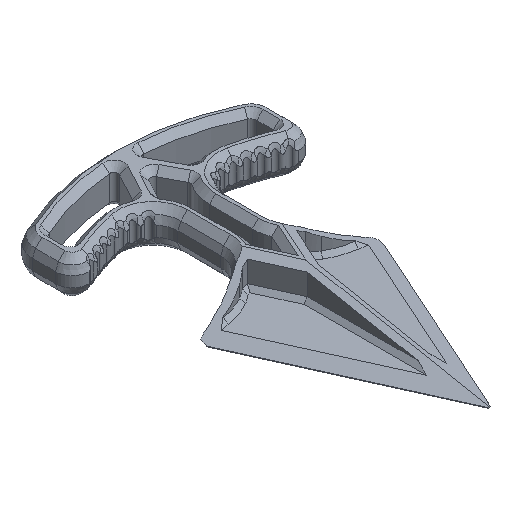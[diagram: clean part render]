
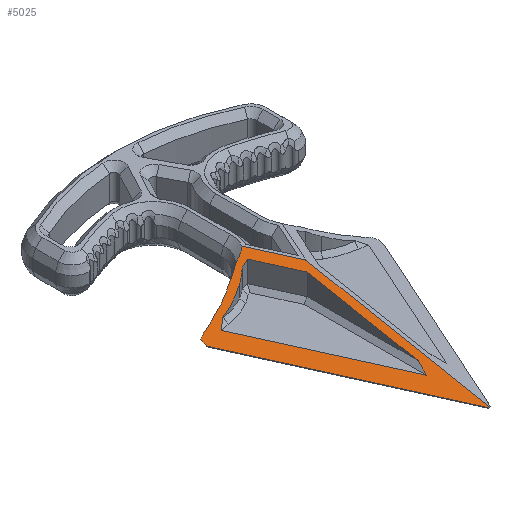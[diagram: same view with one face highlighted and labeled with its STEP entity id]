
A CAD part, isometric view. The second image highlights one B-rep face of the part: STEP entity #5025.
In plain terms, the highlighted planar face has unit normal (-0.385, -0.174, 0.906).
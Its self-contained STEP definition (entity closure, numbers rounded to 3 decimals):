
#60=ELLIPSE('',#5451,39.242,31.462);
#61=ELLIPSE('',#5458,33.593,30.446);
#62=ELLIPSE('',#5460,17.386,15.757);
#63=ELLIPSE('',#5462,13.645,12.367);
#64=ELLIPSE('',#5472,16.739,13.421);
#65=ELLIPSE('',#5475,8.311,6.663);
#66=ELLIPSE('',#5476,16.33,14.522);
#67=ELLIPSE('',#5477,16.084,14.577);
#68=ELLIPSE('',#5478,15.898,14.137);
#94=B_SPLINE_CURVE_WITH_KNOTS('',3,(#7758,#7759,#7760,#7761,#7762,#7763,
#7764,#7765,#7766,#7767,#7768,#7769,#7770),.UNSPECIFIED.,.F.,.F.,(4,3,3,
3,4),(0.053,0.072,0.09,0.104,
0.162),.UNSPECIFIED.);
#96=B_SPLINE_CURVE_WITH_KNOTS('',3,(#7791,#7792,#7793,#7794,#7795,#7796,
#7797),.UNSPECIFIED.,.F.,.F.,(4,3,4),(0.,0.045,0.053),
 .UNSPECIFIED.);
#335=FACE_BOUND('',#926,.T.);
#463=PLANE('',#5474);
#611=FACE_OUTER_BOUND('',#925,.T.);
#925=EDGE_LOOP('',(#3813,#3814,#3815,#3816,#3817,#3818,#3819,#3820,#3821,
#3822,#3823));
#926=EDGE_LOOP('',(#3824,#3825,#3826,#3827,#3828,#3829,#3830,#3831,#3832));
#1325=LINE('',#7068,#1644);
#1443=LINE('',#7509,#1762);
#1469=LINE('',#7636,#1788);
#1475=LINE('',#7653,#1794);
#1477=LINE('',#7657,#1796);
#1478=LINE('',#7659,#1797);
#1482=LINE('',#7669,#1801);
#1489=LINE('',#7700,#1808);
#1491=LINE('',#7809,#1810);
#1644=VECTOR('',#5796,10.);
#1762=VECTOR('',#6242,10.);
#1788=VECTOR('',#6338,10.);
#1794=VECTOR('',#6358,10.);
#1796=VECTOR('',#6362,10.);
#1797=VECTOR('',#6365,10.);
#1801=VECTOR('',#6371,10.);
#1808=VECTOR('',#6386,10.);
#1810=VECTOR('',#6396,10.);
#1970=VERTEX_POINT('',#7065);
#1971=VERTEX_POINT('',#7067);
#2104=VERTEX_POINT('',#7505);
#2106=VERTEX_POINT('',#7508);
#2133=VERTEX_POINT('',#7617);
#2136=VERTEX_POINT('',#7635);
#2137=VERTEX_POINT('',#7639);
#2138=VERTEX_POINT('',#7643);
#2139=VERTEX_POINT('',#7647);
#2140=VERTEX_POINT('',#7651);
#2141=VERTEX_POINT('',#7655);
#2145=VERTEX_POINT('',#7666);
#2146=VERTEX_POINT('',#7668);
#2151=VERTEX_POINT('',#7699);
#2154=VERTEX_POINT('',#7751);
#2156=VERTEX_POINT('',#7757);
#2157=VERTEX_POINT('',#7803);
#2159=VERTEX_POINT('',#7810);
#2160=VERTEX_POINT('',#7812);
#2161=VERTEX_POINT('',#7814);
#2466=EDGE_CURVE('',#1971,#1970,#1325,.T.);
#2678=EDGE_CURVE('',#2106,#2104,#1443,.T.);
#2719=EDGE_CURVE('',#2133,#2104,#60,.T.);
#2726=EDGE_CURVE('',#2106,#2136,#1469,.T.);
#2729=EDGE_CURVE('',#2133,#2137,#61,.T.);
#2731=EDGE_CURVE('',#2137,#2138,#62,.T.);
#2733=EDGE_CURVE('',#2138,#2139,#63,.T.);
#2735=EDGE_CURVE('',#2139,#2140,#1475,.T.);
#2737=EDGE_CURVE('',#2140,#2141,#1477,.T.);
#2738=EDGE_CURVE('',#2141,#2136,#1478,.T.);
#2742=EDGE_CURVE('',#2145,#2146,#1482,.T.);
#2752=EDGE_CURVE('',#2151,#2146,#1489,.T.);
#2758=EDGE_CURVE('',#2154,#2156,#94,.T.);
#2760=EDGE_CURVE('',#2151,#2154,#96,.T.);
#2762=EDGE_CURVE('',#2157,#2156,#64,.T.);
#2765=EDGE_CURVE('',#2145,#1971,#1491,.T.);
#2766=EDGE_CURVE('',#1970,#2159,#65,.T.);
#2767=EDGE_CURVE('',#2159,#2160,#66,.T.);
#2768=EDGE_CURVE('',#2160,#2161,#67,.T.);
#2769=EDGE_CURVE('',#2161,#2157,#68,.T.);
#3813=ORIENTED_EDGE('',*,*,#2742,.F.);
#3814=ORIENTED_EDGE('',*,*,#2765,.T.);
#3815=ORIENTED_EDGE('',*,*,#2466,.T.);
#3816=ORIENTED_EDGE('',*,*,#2766,.T.);
#3817=ORIENTED_EDGE('',*,*,#2767,.T.);
#3818=ORIENTED_EDGE('',*,*,#2768,.T.);
#3819=ORIENTED_EDGE('',*,*,#2769,.T.);
#3820=ORIENTED_EDGE('',*,*,#2762,.T.);
#3821=ORIENTED_EDGE('',*,*,#2758,.F.);
#3822=ORIENTED_EDGE('',*,*,#2760,.F.);
#3823=ORIENTED_EDGE('',*,*,#2752,.T.);
#3824=ORIENTED_EDGE('',*,*,#2738,.T.);
#3825=ORIENTED_EDGE('',*,*,#2726,.F.);
#3826=ORIENTED_EDGE('',*,*,#2678,.T.);
#3827=ORIENTED_EDGE('',*,*,#2719,.F.);
#3828=ORIENTED_EDGE('',*,*,#2729,.T.);
#3829=ORIENTED_EDGE('',*,*,#2731,.T.);
#3830=ORIENTED_EDGE('',*,*,#2733,.T.);
#3831=ORIENTED_EDGE('',*,*,#2735,.T.);
#3832=ORIENTED_EDGE('',*,*,#2737,.T.);
#5025=ADVANCED_FACE('',(#611,#335),#463,.T.);
#5451=AXIS2_PLACEMENT_3D('',#7619,#6322,#6323);
#5458=AXIS2_PLACEMENT_3D('',#7641,#6343,#6344);
#5460=AXIS2_PLACEMENT_3D('',#7645,#6348,#6349);
#5462=AXIS2_PLACEMENT_3D('',#7649,#6353,#6354);
#5472=AXIS2_PLACEMENT_3D('',#7804,#6389,#6390);
#5474=AXIS2_PLACEMENT_3D('',#7808,#6394,#6395);
#5475=AXIS2_PLACEMENT_3D('',#7811,#6397,#6398);
#5476=AXIS2_PLACEMENT_3D('',#7813,#6399,#6400);
#5477=AXIS2_PLACEMENT_3D('',#7815,#6401,#6402);
#5478=AXIS2_PLACEMENT_3D('',#7816,#6403,#6404);
#5796=DIRECTION('',(-0.411,0.911,0.));
#6242=DIRECTION('',(-0.411,0.911,0.));
#6322=DIRECTION('center_axis',(0.385,0.174,-0.906));
#6323=DIRECTION('ref_axis',(0.826,0.373,0.423));
#6338=DIRECTION('',(0.302,0.904,0.302));
#6343=DIRECTION('center_axis',(-0.385,-0.174,0.906));
#6344=DIRECTION('ref_axis',(-0.826,-0.373,-0.423));
#6348=DIRECTION('center_axis',(-0.385,-0.174,0.906));
#6349=DIRECTION('ref_axis',(-0.826,-0.373,-0.423));
#6353=DIRECTION('center_axis',(-0.385,-0.174,0.906));
#6354=DIRECTION('ref_axis',(0.826,0.373,0.423));
#6358=DIRECTION('',(0.879,0.23,0.418));
#6362=DIRECTION('',(0.411,-0.911,0.));
#6365=DIRECTION('',(0.,-0.982,-0.188));
#6371=DIRECTION('',(-0.92,0.,-0.391));
#6386=DIRECTION('',(0.411,-0.911,0.));
#6389=DIRECTION('center_axis',(0.385,0.174,-0.906));
#6390=DIRECTION('ref_axis',(0.826,0.373,0.423));
#6394=DIRECTION('center_axis',(-0.385,-0.174,0.906));
#6395=DIRECTION('ref_axis',(0.92,0.,0.391));
#6396=DIRECTION('',(0.,0.982,0.188));
#6397=DIRECTION('center_axis',(0.385,0.174,-0.906));
#6398=DIRECTION('ref_axis',(0.826,0.373,0.423));
#6399=DIRECTION('center_axis',(0.385,0.174,-0.906));
#6400=DIRECTION('ref_axis',(0.826,0.373,0.423));
#6401=DIRECTION('center_axis',(0.385,0.174,-0.906));
#6402=DIRECTION('ref_axis',(-0.826,-0.373,-0.423));
#6403=DIRECTION('center_axis',(0.385,0.174,-0.906));
#6404=DIRECTION('ref_axis',(0.826,0.373,0.423));
#7065=CARTESIAN_POINT('',(-4.712,-31.269,9.));
#7067=CARTESIAN_POINT('',(0.,-41.71,9.));
#7068=CARTESIAN_POINT('',(1.895,-45.908,9.));
#7505=CARTESIAN_POINT('',(-17.632,-39.134,2.));
#7508=CARTESIAN_POINT('',(-2.4,-72.884,2.));
#7509=CARTESIAN_POINT('',(-10.949,-53.941,2.));
#7617=CARTESIAN_POINT('',(-15.904,-37.75,3.));
#7619=CARTESIAN_POINT('Origin',(-38.221,-14.991,-2.119));
#7635=CARTESIAN_POINT('',(-1.4,-69.886,3.));
#7636=CARTESIAN_POINT('',(3.643,-54.771,8.043));
#7639=CARTESIAN_POINT('',(-15.7,-37.7,3.096));
#7641=CARTESIAN_POINT('Origin',(-23.105,-8.168,5.614));
#7643=CARTESIAN_POINT('',(-9.695,-35.648,6.042));
#7645=CARTESIAN_POINT('Origin',(-17.688,-22.069,5.25));
#7647=CARTESIAN_POINT('',(-7.517,-34.042,7.276));
#7649=CARTESIAN_POINT('Origin',(-15.901,-24.951,5.457));
#7651=CARTESIAN_POINT('',(-5.852,-33.606,8.067));
#7653=CARTESIAN_POINT('',(-9.498,-34.562,6.334));
#7655=CARTESIAN_POINT('',(-1.4,-43.47,8.067));
#7657=CARTESIAN_POINT('',(-1.023,-44.304,8.067));
#7659=CARTESIAN_POINT('',(-1.4,-51.311,6.563));
#7666=CARTESIAN_POINT('',(0.,-85.316,0.635));
#7668=CARTESIAN_POINT('',(-0.309,-85.316,0.504));
#7669=CARTESIAN_POINT('',(-0.147,-85.316,0.572));
#7699=CARTESIAN_POINT('',(-21.104,-39.24,0.504));
#7700=CARTESIAN_POINT('',(-16.823,-48.725,0.504));
#7751=CARTESIAN_POINT('',(-21.037,-38.725,0.631));
#7757=CARTESIAN_POINT('',(-20.873,-37.524,0.931));
#7758=CARTESIAN_POINT('Ctrl Pts',(-21.037,-38.725,0.631));
#7759=CARTESIAN_POINT('Ctrl Pts',(-21.028,-38.663,0.647));
#7760=CARTESIAN_POINT('Ctrl Pts',(-21.019,-38.596,0.664));
#7761=CARTESIAN_POINT('Ctrl Pts',(-21.01,-38.528,0.681));
#7762=CARTESIAN_POINT('Ctrl Pts',(-21.001,-38.461,0.697));
#7763=CARTESIAN_POINT('Ctrl Pts',(-20.992,-38.393,0.714));
#7764=CARTESIAN_POINT('Ctrl Pts',(-20.983,-38.326,0.731));
#7765=CARTESIAN_POINT('Ctrl Pts',(-20.975,-38.271,0.745));
#7766=CARTESIAN_POINT('Ctrl Pts',(-20.968,-38.216,0.758));
#7767=CARTESIAN_POINT('Ctrl Pts',(-20.961,-38.162,0.772));
#7768=CARTESIAN_POINT('Ctrl Pts',(-20.932,-37.949,0.825));
#7769=CARTESIAN_POINT('Ctrl Pts',(-20.903,-37.736,0.878));
#7770=CARTESIAN_POINT('Ctrl Pts',(-20.873,-37.524,0.931));
#7791=CARTESIAN_POINT('Ctrl Pts',(-21.104,-39.24,0.504));
#7792=CARTESIAN_POINT('Ctrl Pts',(-21.086,-39.096,0.54));
#7793=CARTESIAN_POINT('Ctrl Pts',(-21.067,-38.951,0.575));
#7794=CARTESIAN_POINT('Ctrl Pts',(-21.047,-38.807,0.611));
#7795=CARTESIAN_POINT('Ctrl Pts',(-21.044,-38.781,0.618));
#7796=CARTESIAN_POINT('Ctrl Pts',(-21.04,-38.753,0.624));
#7797=CARTESIAN_POINT('Ctrl Pts',(-21.037,-38.725,0.631));
#7803=CARTESIAN_POINT('',(-19.649,-37.047,1.543));
#7804=CARTESIAN_POINT('Origin',(-24.948,-24.716,1.656));
#7808=CARTESIAN_POINT('Origin',(-5.121,-59.031,3.501));
#7809=CARTESIAN_POINT('',(0.,-59.434,5.6));
#7810=CARTESIAN_POINT('',(-7.588,-32.553,7.531));
#7811=CARTESIAN_POINT('Origin',(-8.799,-25.958,8.282));
#7812=CARTESIAN_POINT('',(-10.991,-34.3,5.75));
#7813=CARTESIAN_POINT('Origin',(-15.894,-20.63,6.288));
#7814=CARTESIAN_POINT('',(-16.028,-36.172,3.25));
#7815=CARTESIAN_POINT('Origin',(-18.5,-21.806,4.955));
#7816=CARTESIAN_POINT('Origin',(-21.037,-22.951,3.657));
